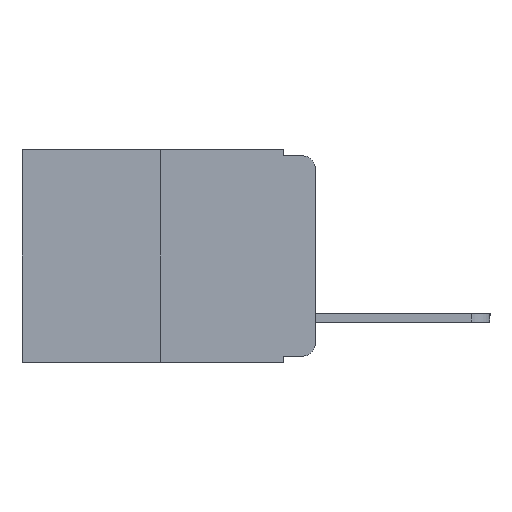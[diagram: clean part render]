
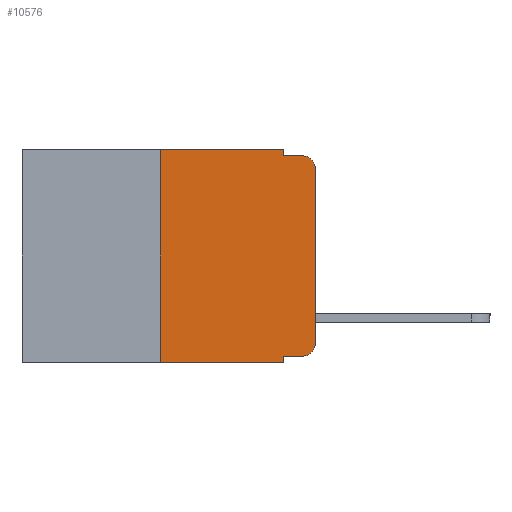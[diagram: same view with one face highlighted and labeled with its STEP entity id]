
A CAD part, left-side view. The second image highlights one B-rep face of the part: STEP entity #10576.
In plain terms, the highlighted planar face has unit normal (-1, 0, 0).
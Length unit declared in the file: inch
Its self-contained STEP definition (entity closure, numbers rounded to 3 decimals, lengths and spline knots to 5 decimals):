
#40 = VECTOR ( 'NONE', #2824, 39.37008 ) ;
#46 = ORIENTED_EDGE ( 'NONE', *, *, #17097, .T. ) ;
#80 = VERTEX_POINT ( 'NONE', #8556 ) ;
#195 = CARTESIAN_POINT ( 'NONE',  ( 0., 0.051, 0. ) ) ;
#568 = ORIENTED_EDGE ( 'NONE', *, *, #5782, .T. ) ;
#625 = VECTOR ( 'NONE', #17184, 39.37008 ) ;
#637 = DIRECTION ( 'NONE',  ( -1., 0., 0. ) ) ;
#822 = CARTESIAN_POINT ( 'NONE',  ( 0., 0.051, -0.01 ) ) ;
#1007 = VERTEX_POINT ( 'NONE', #7033 ) ;
#1789 = LINE ( 'NONE', #22853, #12137 ) ;
#1812 = CARTESIAN_POINT ( 'NONE',  ( 0., 0., 0. ) ) ;
#1854 = VECTOR ( 'NONE', #2224, 39.37008 ) ;
#2083 = EDGE_CURVE ( 'NONE', #2611, #14438, #1789, .T. ) ;
#2224 = DIRECTION ( 'NONE',  ( 0., 0., -1. ) ) ;
#2254 = AXIS2_PLACEMENT_3D ( 'NONE', #18768, #22464, #11247 ) ;
#2416 = ORIENTED_EDGE ( 'NONE', *, *, #14629, .F. ) ;
#2611 = VERTEX_POINT ( 'NONE', #21883 ) ;
#2824 = DIRECTION ( 'NONE',  ( 0., -1., 0. ) ) ;
#2889 = DIRECTION ( 'NONE',  ( 0., -1., 0. ) ) ;
#3147 = EDGE_CURVE ( 'NONE', #80, #15685, #17715, .T. ) ;
#3452 = PLANE ( 'NONE',  #2254 ) ;
#3884 = ORIENTED_EDGE ( 'NONE', *, *, #10788, .F. ) ;
#4014 = LINE ( 'NONE', #21775, #9789 ) ;
#4309 = EDGE_CURVE ( 'NONE', #1007, #12131, #20468, .T. ) ;
#5239 = CARTESIAN_POINT ( 'NONE',  ( 0., 0.473, -0.343 ) ) ;
#5782 = EDGE_CURVE ( 'NONE', #1007, #80, #4014, .T. ) ;
#6068 = DIRECTION ( 'NONE',  ( -1., 0., 0. ) ) ;
#6525 = VECTOR ( 'NONE', #22649, 39.37008 ) ;
#6585 = ORIENTED_EDGE ( 'NONE', *, *, #2083, .F. ) ;
#6700 = CARTESIAN_POINT ( 'NONE',  ( 0., 0.25, -0.343 ) ) ;
#7033 = CARTESIAN_POINT ( 'NONE',  ( 0., 0.051, -0.333 ) ) ;
#7264 = LINE ( 'NONE', #12132, #21129 ) ;
#7595 = CARTESIAN_POINT ( 'NONE',  ( 0., 0.051, 0. ) ) ;
#7753 = ORIENTED_EDGE ( 'NONE', *, *, #11111, .T. ) ;
#8178 = CARTESIAN_POINT ( 'NONE',  ( 0., 0., -0.03 ) ) ;
#8556 = CARTESIAN_POINT ( 'NONE',  ( 0., 0.02, -0.333 ) ) ;
#9641 = DIRECTION ( 'NONE',  ( 0., 0., -1. ) ) ;
#9664 = ORIENTED_EDGE ( 'NONE', *, *, #4309, .F. ) ;
#9789 = VECTOR ( 'NONE', #23635, 39.37008 ) ;
#10117 = AXIS2_PLACEMENT_3D ( 'NONE', #21937, #6068, #9641 ) ;
#10576 = ADVANCED_FACE ( 'NONE', ( #22430 ), #3452, .F. ) ;
#10788 = EDGE_CURVE ( 'NONE', #14438, #13019, #17177, .T. ) ;
#11111 = EDGE_CURVE ( 'NONE', #13228, #12131, #15130, .T. ) ;
#11161 = AXIS2_PLACEMENT_3D ( 'NONE', #12317, #637, #14247 ) ;
#11247 = DIRECTION ( 'NONE',  ( 0., 0., -1. ) ) ;
#11680 = ORIENTED_EDGE ( 'NONE', *, *, #19614, .T. ) ;
#12131 = VERTEX_POINT ( 'NONE', #17780 ) ;
#12132 = CARTESIAN_POINT ( 'NONE',  ( 0., 0.25, 0. ) ) ;
#12137 = VECTOR ( 'NONE', #2889, 39.37008 ) ;
#12317 = CARTESIAN_POINT ( 'NONE',  ( 0., 0.02, -0.03 ) ) ;
#13019 = VERTEX_POINT ( 'NONE', #24079 ) ;
#13228 = VERTEX_POINT ( 'NONE', #6700 ) ;
#13367 = EDGE_CURVE ( 'NONE', #13228, #2611, #7264, .T. ) ;
#14058 = DIRECTION ( 'NONE',  ( 0., 0., 1. ) ) ;
#14247 = DIRECTION ( 'NONE',  ( 0., 0., -1. ) ) ;
#14438 = VERTEX_POINT ( 'NONE', #15627 ) ;
#14629 = EDGE_CURVE ( 'NONE', #13019, #15484, #15525, .T. ) ;
#15130 = LINE ( 'NONE', #5239, #19522 ) ;
#15484 = VERTEX_POINT ( 'NONE', #16803 ) ;
#15525 = LINE ( 'NONE', #822, #40 ) ;
#15627 = CARTESIAN_POINT ( 'NONE',  ( 0., 0.051, 0. ) ) ;
#15685 = VERTEX_POINT ( 'NONE', #22432 ) ;
#15953 = VERTEX_POINT ( 'NONE', #8178 ) ;
#16803 = CARTESIAN_POINT ( 'NONE',  ( 0., 0.02, -0.01 ) ) ;
#17097 = EDGE_CURVE ( 'NONE', #15953, #15484, #22823, .T. ) ;
#17177 = LINE ( 'NONE', #195, #1854 ) ;
#17184 = DIRECTION ( 'NONE',  ( 0., 0., 1. ) ) ;
#17715 = CIRCLE ( 'NONE', #10117, 0.02 ) ;
#17780 = CARTESIAN_POINT ( 'NONE',  ( 0., 0.051, -0.343 ) ) ;
#18768 = CARTESIAN_POINT ( 'NONE',  ( 0., 0.473, 0. ) ) ;
#18949 = EDGE_LOOP ( 'NONE', ( #11680, #46, #2416, #3884, #6585, #24639, #7753, #9664, #568, #19411 ) ) ;
#19411 = ORIENTED_EDGE ( 'NONE', *, *, #3147, .T. ) ;
#19522 = VECTOR ( 'NONE', #24078, 39.37008 ) ;
#19614 = EDGE_CURVE ( 'NONE', #15685, #15953, #21000, .T. ) ;
#20468 = LINE ( 'NONE', #7595, #6525 ) ;
#21000 = LINE ( 'NONE', #1812, #625 ) ;
#21129 = VECTOR ( 'NONE', #14058, 39.37008 ) ;
#21775 = CARTESIAN_POINT ( 'NONE',  ( 0., 0.051, -0.333 ) ) ;
#21883 = CARTESIAN_POINT ( 'NONE',  ( 0., 0.25, 0. ) ) ;
#21937 = CARTESIAN_POINT ( 'NONE',  ( 0., 0.02, -0.313 ) ) ;
#22430 = FACE_OUTER_BOUND ( 'NONE', #18949, .T. ) ;
#22432 = CARTESIAN_POINT ( 'NONE',  ( 0., 0., -0.313 ) ) ;
#22464 = DIRECTION ( 'NONE',  ( 1., 0., 0. ) ) ;
#22649 = DIRECTION ( 'NONE',  ( 0., 0., -1. ) ) ;
#22823 = CIRCLE ( 'NONE', #11161, 0.02 ) ;
#22853 = CARTESIAN_POINT ( 'NONE',  ( 0., 0.473, 0. ) ) ;
#23635 = DIRECTION ( 'NONE',  ( 0., -1., 0. ) ) ;
#24078 = DIRECTION ( 'NONE',  ( 0., -1., 0. ) ) ;
#24079 = CARTESIAN_POINT ( 'NONE',  ( 0., 0.051, -0.01 ) ) ;
#24639 = ORIENTED_EDGE ( 'NONE', *, *, #13367, .F. ) ;
